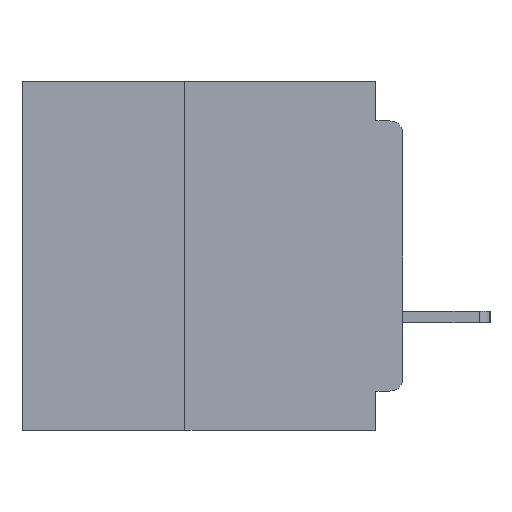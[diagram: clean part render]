
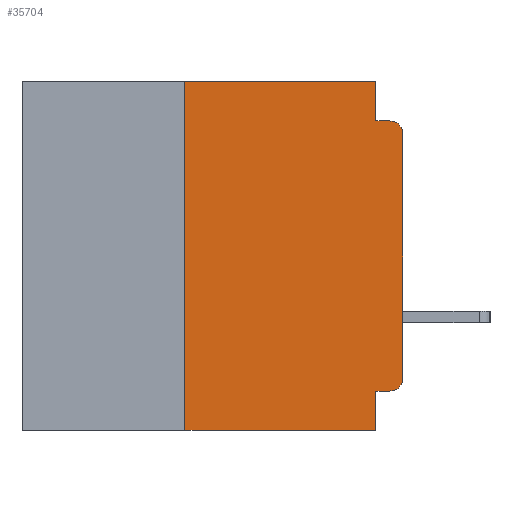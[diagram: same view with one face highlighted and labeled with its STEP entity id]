
A CAD part, left-side view. The second image highlights one B-rep face of the part: STEP entity #35704.
In plain terms, the highlighted planar face has unit normal (-1, 0, 0).
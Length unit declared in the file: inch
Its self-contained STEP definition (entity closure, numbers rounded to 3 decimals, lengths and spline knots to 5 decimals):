
#274 = CARTESIAN_POINT ( 'NONE',  ( 0., 0.25, -0.4 ) ) ;
#440 = VECTOR ( 'NONE', #35306, 39.37008 ) ;
#507 = LINE ( 'NONE', #9262, #7062 ) ;
#931 = ORIENTED_EDGE ( 'NONE', *, *, #32505, .F. ) ;
#1543 = DIRECTION ( 'NONE',  ( 0., 0., -1. ) ) ;
#1920 = LINE ( 'NONE', #274, #22502 ) ;
#2179 = CARTESIAN_POINT ( 'NONE',  ( 0., 0.031, -0.045 ) ) ;
#2438 = CARTESIAN_POINT ( 'NONE',  ( 0., 0.437, 0. ) ) ;
#3564 = EDGE_CURVE ( 'NONE', #20307, #25468, #5192, .T. ) ;
#3826 = LINE ( 'NONE', #2438, #31678 ) ;
#3887 = EDGE_CURVE ( 'NONE', #4119, #5747, #25260, .T. ) ;
#3990 = LINE ( 'NONE', #13409, #18033 ) ;
#4119 = VERTEX_POINT ( 'NONE', #29213 ) ;
#5192 = CIRCLE ( 'NONE', #6425, 0.015 ) ;
#5634 = VERTEX_POINT ( 'NONE', #15594 ) ;
#5740 = CARTESIAN_POINT ( 'NONE',  ( 0., 0., -0.06 ) ) ;
#5747 = VERTEX_POINT ( 'NONE', #29752 ) ;
#5877 = DIRECTION ( 'NONE',  ( 0., 0., 1. ) ) ;
#6425 = AXIS2_PLACEMENT_3D ( 'NONE', #14351, #12093, #1543 ) ;
#7062 = VECTOR ( 'NONE', #25869, 39.37008 ) ;
#7492 = VERTEX_POINT ( 'NONE', #21825 ) ;
#7506 = EDGE_CURVE ( 'NONE', #5634, #7492, #3990, .T. ) ;
#7514 = PLANE ( 'NONE',  #10458 ) ;
#7814 = ORIENTED_EDGE ( 'NONE', *, *, #19469, .T. ) ;
#8659 = ORIENTED_EDGE ( 'NONE', *, *, #10350, .F. ) ;
#8856 = EDGE_CURVE ( 'NONE', #4119, #5634, #32231, .T. ) ;
#9262 = CARTESIAN_POINT ( 'NONE',  ( 0., 0.031, 0. ) ) ;
#9838 = VERTEX_POINT ( 'NONE', #26877 ) ;
#9976 = CARTESIAN_POINT ( 'NONE',  ( 0., 0.015, -0.045 ) ) ;
#10069 = VECTOR ( 'NONE', #33049, 39.37008 ) ;
#10350 = EDGE_CURVE ( 'NONE', #14001, #13422, #3826, .T. ) ;
#10458 = AXIS2_PLACEMENT_3D ( 'NONE', #18710, #32570, #16005 ) ;
#11801 = ORIENTED_EDGE ( 'NONE', *, *, #8856, .F. ) ;
#12093 = DIRECTION ( 'NONE',  ( -1., 0., 0. ) ) ;
#12657 = ORIENTED_EDGE ( 'NONE', *, *, #18662, .F. ) ;
#13188 = FACE_OUTER_BOUND ( 'NONE', #16411, .T. ) ;
#13255 = AXIS2_PLACEMENT_3D ( 'NONE', #21827, #21743, #20886 ) ;
#13409 = CARTESIAN_POINT ( 'NONE',  ( 0., 0.031, -0.4 ) ) ;
#13422 = VERTEX_POINT ( 'NONE', #23398 ) ;
#14001 = VERTEX_POINT ( 'NONE', #20342 ) ;
#14351 = CARTESIAN_POINT ( 'NONE',  ( 0., 0.015, -0.06 ) ) ;
#15026 = CARTESIAN_POINT ( 'NONE',  ( 0., 0., -0.045 ) ) ;
#15043 = LINE ( 'NONE', #17155, #20728 ) ;
#15361 = LINE ( 'NONE', #32662, #440 ) ;
#15594 = CARTESIAN_POINT ( 'NONE',  ( 0., 0.031, -0.355 ) ) ;
#16005 = DIRECTION ( 'NONE',  ( 0., 0., -1. ) ) ;
#16411 = EDGE_LOOP ( 'NONE', ( #28156, #35519, #931, #12657, #8659, #18572, #7814, #34108, #11801, #22550 ) ) ;
#17155 = CARTESIAN_POINT ( 'NONE',  ( 0., 0., 0. ) ) ;
#17837 = DIRECTION ( 'NONE',  ( 0., -1., 0. ) ) ;
#18017 = EDGE_CURVE ( 'NONE', #5747, #20307, #15043, .T. ) ;
#18033 = VECTOR ( 'NONE', #27369, 39.37008 ) ;
#18572 = ORIENTED_EDGE ( 'NONE', *, *, #31168, .F. ) ;
#18662 = EDGE_CURVE ( 'NONE', #13422, #20138, #507, .T. ) ;
#18710 = CARTESIAN_POINT ( 'NONE',  ( 0., 0.437, 0. ) ) ;
#19469 = EDGE_CURVE ( 'NONE', #9838, #7492, #15361, .T. ) ;
#20138 = VERTEX_POINT ( 'NONE', #2179 ) ;
#20307 = VERTEX_POINT ( 'NONE', #5740 ) ;
#20342 = CARTESIAN_POINT ( 'NONE',  ( 0., 0.25, 0. ) ) ;
#20728 = VECTOR ( 'NONE', #5877, 39.37008 ) ;
#20886 = DIRECTION ( 'NONE',  ( 0., 0., -1. ) ) ;
#21160 = LINE ( 'NONE', #15026, #34927 ) ;
#21743 = DIRECTION ( 'NONE',  ( -1., 0., 0. ) ) ;
#21825 = CARTESIAN_POINT ( 'NONE',  ( 0., 0.031, -0.4 ) ) ;
#21827 = CARTESIAN_POINT ( 'NONE',  ( 0., 0.015, -0.34 ) ) ;
#22502 = VECTOR ( 'NONE', #22652, 39.37008 ) ;
#22550 = ORIENTED_EDGE ( 'NONE', *, *, #3887, .T. ) ;
#22652 = DIRECTION ( 'NONE',  ( 0., 0., 1. ) ) ;
#23398 = CARTESIAN_POINT ( 'NONE',  ( 0., 0.031, 0. ) ) ;
#24827 = DIRECTION ( 'NONE',  ( 0., -1., 0. ) ) ;
#25260 = CIRCLE ( 'NONE', #13255, 0.015 ) ;
#25468 = VERTEX_POINT ( 'NONE', #9976 ) ;
#25869 = DIRECTION ( 'NONE',  ( 0., 0., -1. ) ) ;
#26877 = CARTESIAN_POINT ( 'NONE',  ( 0., 0.25, -0.4 ) ) ;
#27369 = DIRECTION ( 'NONE',  ( 0., 0., -1. ) ) ;
#28156 = ORIENTED_EDGE ( 'NONE', *, *, #18017, .T. ) ;
#29213 = CARTESIAN_POINT ( 'NONE',  ( 0., 0.015, -0.355 ) ) ;
#29752 = CARTESIAN_POINT ( 'NONE',  ( 0., 0., -0.34 ) ) ;
#30278 = CARTESIAN_POINT ( 'NONE',  ( 0., 0., -0.355 ) ) ;
#31168 = EDGE_CURVE ( 'NONE', #9838, #14001, #1920, .T. ) ;
#31678 = VECTOR ( 'NONE', #24827, 39.37008 ) ;
#32231 = LINE ( 'NONE', #30278, #10069 ) ;
#32505 = EDGE_CURVE ( 'NONE', #20138, #25468, #21160, .T. ) ;
#32570 = DIRECTION ( 'NONE',  ( 1., 0., 0. ) ) ;
#32662 = CARTESIAN_POINT ( 'NONE',  ( 0., 0.437, -0.4 ) ) ;
#33049 = DIRECTION ( 'NONE',  ( 0., 1., 0. ) ) ;
#34108 = ORIENTED_EDGE ( 'NONE', *, *, #7506, .F. ) ;
#34927 = VECTOR ( 'NONE', #17837, 39.37008 ) ;
#35306 = DIRECTION ( 'NONE',  ( 0., -1., 0. ) ) ;
#35519 = ORIENTED_EDGE ( 'NONE', *, *, #3564, .T. ) ;
#35704 = ADVANCED_FACE ( 'NONE', ( #13188 ), #7514, .F. ) ;
